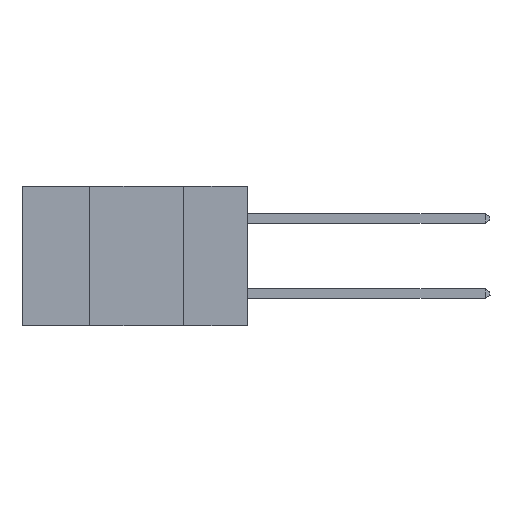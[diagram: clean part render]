
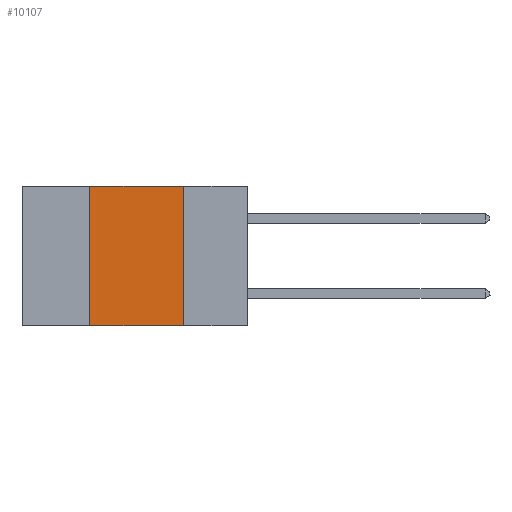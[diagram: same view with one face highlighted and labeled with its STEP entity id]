
A CAD part, left-side view. The second image highlights one B-rep face of the part: STEP entity #10107.
In plain terms, the highlighted planar face has unit normal (-1, 0, 0).
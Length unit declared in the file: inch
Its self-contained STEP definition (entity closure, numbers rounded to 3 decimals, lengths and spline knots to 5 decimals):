
#1027 = DIRECTION ( 'NONE',  ( 0., 0., 1. ) ) ;
#1317 = VERTEX_POINT ( 'NONE', #5051 ) ;
#2301 = DIRECTION ( 'NONE',  ( 0., -1., 0. ) ) ;
#2756 = LINE ( 'NONE', #13828, #12106 ) ;
#2787 = EDGE_CURVE ( 'NONE', #4856, #1317, #8460, .T. ) ;
#3290 = AXIS2_PLACEMENT_3D ( 'NONE', #10483, #3413, #3474 ) ;
#3413 = DIRECTION ( 'NONE',  ( 1., 0., 0. ) ) ;
#3474 = DIRECTION ( 'NONE',  ( 0., 0., -1. ) ) ;
#4403 = VECTOR ( 'NONE', #8792, 39.37008 ) ;
#4730 = EDGE_CURVE ( 'NONE', #10569, #1317, #12038, .T. ) ;
#4812 = VECTOR ( 'NONE', #9297, 39.37008 ) ;
#4856 = VERTEX_POINT ( 'NONE', #7499 ) ;
#5051 = CARTESIAN_POINT ( 'NONE',  ( 0., 0.17, -0.37 ) ) ;
#6504 = CARTESIAN_POINT ( 'NONE',  ( 0., 0.6, 0. ) ) ;
#6777 = EDGE_CURVE ( 'NONE', #10569, #12394, #2756, .T. ) ;
#7499 = CARTESIAN_POINT ( 'NONE',  ( 0., 0.17, 0. ) ) ;
#7904 = EDGE_CURVE ( 'NONE', #12394, #4856, #14491, .T. ) ;
#7911 = CARTESIAN_POINT ( 'NONE',  ( 0., 0.17, 0. ) ) ;
#8021 = CARTESIAN_POINT ( 'NONE',  ( 0., 0.42, -0.37 ) ) ;
#8258 = PLANE ( 'NONE',  #3290 ) ;
#8460 = LINE ( 'NONE', #7911, #4812 ) ;
#8504 = EDGE_LOOP ( 'NONE', ( #9492, #11595, #12606, #10003 ) ) ;
#8792 = DIRECTION ( 'NONE',  ( 0., -1., 0. ) ) ;
#9105 = CARTESIAN_POINT ( 'NONE',  ( 0., 0.42, 0. ) ) ;
#9297 = DIRECTION ( 'NONE',  ( 0., 0., -1. ) ) ;
#9492 = ORIENTED_EDGE ( 'NONE', *, *, #2787, .F. ) ;
#10003 = ORIENTED_EDGE ( 'NONE', *, *, #4730, .T. ) ;
#10107 = ADVANCED_FACE ( 'NONE', ( #10198 ), #8258, .F. ) ;
#10198 = FACE_OUTER_BOUND ( 'NONE', #8504, .T. ) ;
#10483 = CARTESIAN_POINT ( 'NONE',  ( 0., 0.6, 0. ) ) ;
#10569 = VERTEX_POINT ( 'NONE', #8021 ) ;
#11595 = ORIENTED_EDGE ( 'NONE', *, *, #7904, .F. ) ;
#12005 = CARTESIAN_POINT ( 'NONE',  ( 0., 0.6, -0.37 ) ) ;
#12038 = LINE ( 'NONE', #12005, #15141 ) ;
#12106 = VECTOR ( 'NONE', #1027, 39.37008 ) ;
#12394 = VERTEX_POINT ( 'NONE', #9105 ) ;
#12606 = ORIENTED_EDGE ( 'NONE', *, *, #6777, .F. ) ;
#13828 = CARTESIAN_POINT ( 'NONE',  ( 0., 0.42, 0. ) ) ;
#14491 = LINE ( 'NONE', #6504, #4403 ) ;
#15141 = VECTOR ( 'NONE', #2301, 39.37008 ) ;
